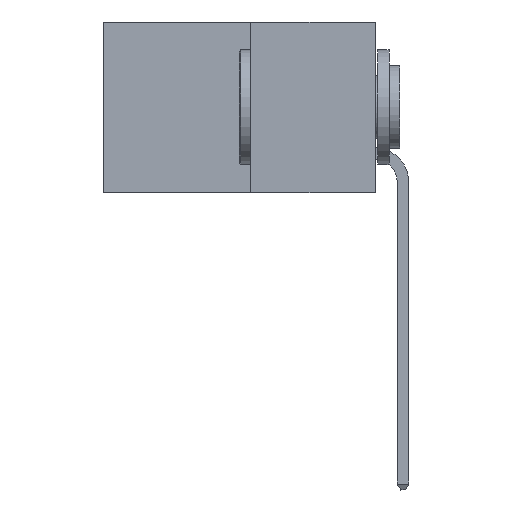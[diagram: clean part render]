
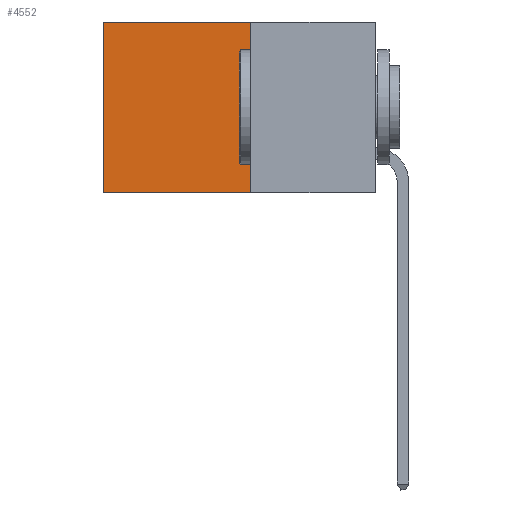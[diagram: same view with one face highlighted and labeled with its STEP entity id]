
A CAD part, left-side view. The second image highlights one B-rep face of the part: STEP entity #4552.
In plain terms, the highlighted planar face has unit normal (-1, 0, 0).
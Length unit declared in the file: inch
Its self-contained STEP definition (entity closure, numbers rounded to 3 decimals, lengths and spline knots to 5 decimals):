
#824 = CARTESIAN_POINT ( 'NONE',  ( 0.277, 0.59, -0.37 ) ) ;
#1234 = CARTESIAN_POINT ( 'NONE',  ( 0.277, 0.27, -0.37 ) ) ;
#2190 = VERTEX_POINT ( 'NONE', #12743 ) ;
#2638 = DIRECTION ( 'NONE',  ( 0., 1., 0. ) ) ;
#3810 = AXIS2_PLACEMENT_3D ( 'NONE', #11825, #11568, #11521 ) ;
#3941 = DIRECTION ( 'NONE',  ( 0., 0., -1. ) ) ;
#4552 = ADVANCED_FACE ( 'NONE', ( #9409 ), #11617, .F. ) ;
#5146 = LINE ( 'NONE', #1234, #17346 ) ;
#5635 = VERTEX_POINT ( 'NONE', #14967 ) ;
#5925 = VECTOR ( 'NONE', #2638, 39.37008 ) ;
#6227 = CARTESIAN_POINT ( 'NONE',  ( 0.277, 0.27, -0.37 ) ) ;
#6423 = ORIENTED_EDGE ( 'NONE', *, *, #14534, .T. ) ;
#7222 = CARTESIAN_POINT ( 'NONE',  ( 0.277, 0.59, -0.37 ) ) ;
#8683 = VECTOR ( 'NONE', #16252, 39.37008 ) ;
#8986 = EDGE_CURVE ( 'NONE', #5635, #11714, #11532, .T. ) ;
#9409 = FACE_OUTER_BOUND ( 'NONE', #18235, .T. ) ;
#9603 = DIRECTION ( 'NONE',  ( 0., 0., -1. ) ) ;
#9975 = ORIENTED_EDGE ( 'NONE', *, *, #8986, .T. ) ;
#10131 = ORIENTED_EDGE ( 'NONE', *, *, #13146, .F. ) ;
#11521 = DIRECTION ( 'NONE',  ( 0., 0., -1. ) ) ;
#11532 = LINE ( 'NONE', #7222, #13849 ) ;
#11568 = DIRECTION ( 'NONE',  ( 1., 0., 0. ) ) ;
#11617 = PLANE ( 'NONE',  #3810 ) ;
#11714 = VERTEX_POINT ( 'NONE', #824 ) ;
#11825 = CARTESIAN_POINT ( 'NONE',  ( 0.277, 0.27, -0.37 ) ) ;
#12559 = CARTESIAN_POINT ( 'NONE',  ( 0.277, 0.27, -0.37 ) ) ;
#12743 = CARTESIAN_POINT ( 'NONE',  ( 0.277, 0.27, 0. ) ) ;
#12879 = CARTESIAN_POINT ( 'NONE',  ( 0.277, 0.27, 0. ) ) ;
#13146 = EDGE_CURVE ( 'NONE', #13256, #11714, #13678, .T. ) ;
#13256 = VERTEX_POINT ( 'NONE', #6227 ) ;
#13603 = LINE ( 'NONE', #12879, #8683 ) ;
#13678 = LINE ( 'NONE', #12559, #5925 ) ;
#13849 = VECTOR ( 'NONE', #3941, 39.37008 ) ;
#14534 = EDGE_CURVE ( 'NONE', #2190, #5635, #13603, .T. ) ;
#14967 = CARTESIAN_POINT ( 'NONE',  ( 0.277, 0.59, 0. ) ) ;
#16252 = DIRECTION ( 'NONE',  ( 0., 1., 0. ) ) ;
#16873 = ORIENTED_EDGE ( 'NONE', *, *, #20162, .F. ) ;
#17346 = VECTOR ( 'NONE', #9603, 39.37008 ) ;
#18235 = EDGE_LOOP ( 'NONE', ( #9975, #10131, #16873, #6423 ) ) ;
#20162 = EDGE_CURVE ( 'NONE', #2190, #13256, #5146, .T. ) ;
